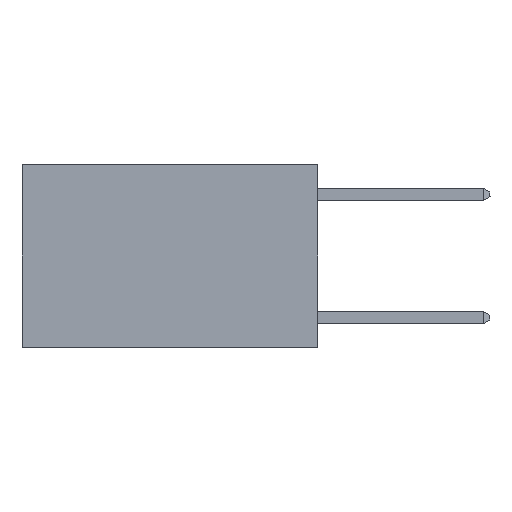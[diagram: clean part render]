
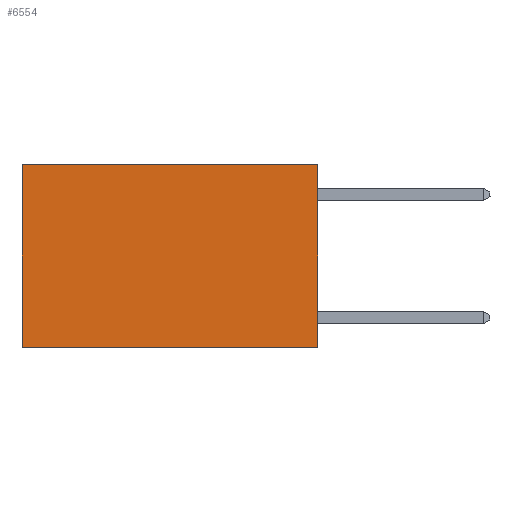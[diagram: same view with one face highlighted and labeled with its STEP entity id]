
A CAD part, left-side view. The second image highlights one B-rep face of the part: STEP entity #6554.
In plain terms, the highlighted planar face has unit normal (-1, 0, 0).
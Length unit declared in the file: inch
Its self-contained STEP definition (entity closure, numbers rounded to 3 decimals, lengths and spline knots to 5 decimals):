
#238 = LINE ( 'NONE', #16181, #3708 ) ;
#1209 = LINE ( 'NONE', #9395, #11118 ) ;
#1650 = DIRECTION ( 'NONE',  ( 0., 1., 0. ) ) ;
#2018 = ORIENTED_EDGE ( 'NONE', *, *, #12762, .T. ) ;
#2245 = EDGE_CURVE ( 'NONE', #8693, #4918, #10972, .T. ) ;
#2795 = EDGE_CURVE ( 'NONE', #5691, #4918, #238, .T. ) ;
#3405 = DIRECTION ( 'NONE',  ( 0., 0., -1. ) ) ;
#3613 = CARTESIAN_POINT ( 'NONE',  ( 0.2625, 0.6, 0. ) ) ;
#3708 = VECTOR ( 'NONE', #16212, 39.37008 ) ;
#3863 = ORIENTED_EDGE ( 'NONE', *, *, #2795, .F. ) ;
#4303 = ORIENTED_EDGE ( 'NONE', *, *, #2245, .T. ) ;
#4339 = CARTESIAN_POINT ( 'NONE',  ( 0.2625, 0., 0. ) ) ;
#4806 = FACE_OUTER_BOUND ( 'NONE', #15014, .T. ) ;
#4918 = VERTEX_POINT ( 'NONE', #10764 ) ;
#5153 = LINE ( 'NONE', #9236, #11179 ) ;
#5255 = VERTEX_POINT ( 'NONE', #16646 ) ;
#5634 = DIRECTION ( 'NONE',  ( 1., 0., 0. ) ) ;
#5691 = VERTEX_POINT ( 'NONE', #12237 ) ;
#6554 = ADVANCED_FACE ( 'NONE', ( #4806 ), #12049, .F. ) ;
#6729 = DIRECTION ( 'NONE',  ( 0., 0., -1. ) ) ;
#7123 = AXIS2_PLACEMENT_3D ( 'NONE', #4339, #5634, #14703 ) ;
#7551 = VECTOR ( 'NONE', #3405, 39.37008 ) ;
#7676 = EDGE_CURVE ( 'NONE', #5255, #5691, #5153, .T. ) ;
#8693 = VERTEX_POINT ( 'NONE', #13793 ) ;
#9235 = ORIENTED_EDGE ( 'NONE', *, *, #7676, .F. ) ;
#9236 = CARTESIAN_POINT ( 'NONE',  ( 0.2625, 0., 0. ) ) ;
#9395 = CARTESIAN_POINT ( 'NONE',  ( 0.2625, 0., 0. ) ) ;
#10764 = CARTESIAN_POINT ( 'NONE',  ( 0.2625, 0.6, -0.37 ) ) ;
#10972 = LINE ( 'NONE', #3613, #7551 ) ;
#11118 = VECTOR ( 'NONE', #1650, 39.37008 ) ;
#11179 = VECTOR ( 'NONE', #6729, 39.37008 ) ;
#12049 = PLANE ( 'NONE',  #7123 ) ;
#12237 = CARTESIAN_POINT ( 'NONE',  ( 0.2625, 0., -0.37 ) ) ;
#12762 = EDGE_CURVE ( 'NONE', #5255, #8693, #1209, .T. ) ;
#13793 = CARTESIAN_POINT ( 'NONE',  ( 0.2625, 0.6, 0. ) ) ;
#14703 = DIRECTION ( 'NONE',  ( 0., 0., -1. ) ) ;
#15014 = EDGE_LOOP ( 'NONE', ( #4303, #3863, #9235, #2018 ) ) ;
#16181 = CARTESIAN_POINT ( 'NONE',  ( 0.2625, 0., -0.37 ) ) ;
#16212 = DIRECTION ( 'NONE',  ( 0., 1., 0. ) ) ;
#16646 = CARTESIAN_POINT ( 'NONE',  ( 0.2625, 0., 0. ) ) ;
